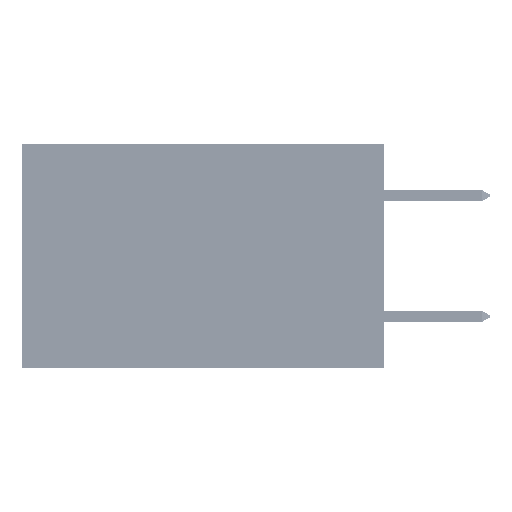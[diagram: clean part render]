
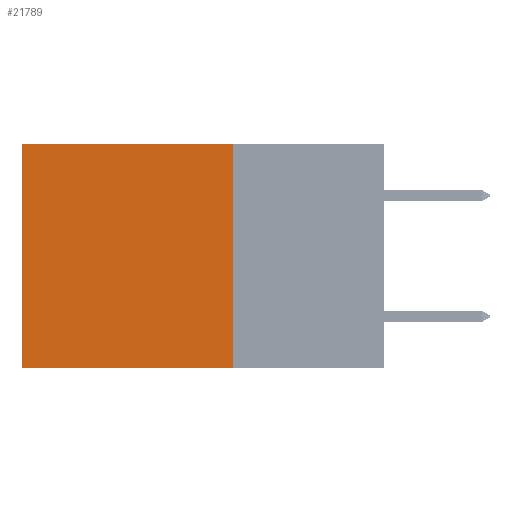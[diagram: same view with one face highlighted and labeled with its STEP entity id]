
A CAD part, left-side view. The second image highlights one B-rep face of the part: STEP entity #21789.
In plain terms, the highlighted planar face has unit normal (-1, 0, 0).
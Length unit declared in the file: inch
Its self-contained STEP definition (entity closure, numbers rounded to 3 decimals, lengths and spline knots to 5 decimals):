
#695 = ORIENTED_EDGE ( 'NONE', *, *, #42039, .T. ) ;
#1182 = VECTOR ( 'NONE', #9158, 39.37008 ) ;
#1398 = DIRECTION ( 'NONE',  ( 0., 1., 0. ) ) ;
#4452 = ORIENTED_EDGE ( 'NONE', *, *, #6993, .T. ) ;
#5292 = EDGE_CURVE ( 'NONE', #37169, #43508, #27434, .T. ) ;
#5573 = CARTESIAN_POINT ( 'NONE',  ( 0.2875, 0.25, 0. ) ) ;
#5742 = CARTESIAN_POINT ( 'NONE',  ( 0.2875, 0.25, 0. ) ) ;
#6723 = ORIENTED_EDGE ( 'NONE', *, *, #9416, .F. ) ;
#6993 = EDGE_CURVE ( 'NONE', #26703, #14465, #40642, .T. ) ;
#8527 = VECTOR ( 'NONE', #34752, 39.37008 ) ;
#8702 = DIRECTION ( 'NONE',  ( 0., 0., -1. ) ) ;
#8930 = LINE ( 'NONE', #22814, #25578 ) ;
#9158 = DIRECTION ( 'NONE',  ( 0., 0., -1. ) ) ;
#9416 = EDGE_CURVE ( 'NONE', #26703, #37169, #10590, .T. ) ;
#9745 = CARTESIAN_POINT ( 'NONE',  ( 0.2875, 0.25, -0.37 ) ) ;
#10570 = CARTESIAN_POINT ( 'NONE',  ( 0.2875, 0.6, 0. ) ) ;
#10590 = LINE ( 'NONE', #5573, #1182 ) ;
#12317 = VECTOR ( 'NONE', #1398, 39.37008 ) ;
#14465 = VERTEX_POINT ( 'NONE', #10570 ) ;
#20741 = ORIENTED_EDGE ( 'NONE', *, *, #5292, .F. ) ;
#21789 = ADVANCED_FACE ( 'NONE', ( #25027 ), #40375, .F. ) ;
#22814 = CARTESIAN_POINT ( 'NONE',  ( 0.2875, 0.6, 0. ) ) ;
#25027 = FACE_OUTER_BOUND ( 'NONE', #33649, .T. ) ;
#25578 = VECTOR ( 'NONE', #8702, 39.37008 ) ;
#26131 = DIRECTION ( 'NONE',  ( 1., 0., 0. ) ) ;
#26266 = CARTESIAN_POINT ( 'NONE',  ( 0.2875, 0.25, 0. ) ) ;
#26703 = VERTEX_POINT ( 'NONE', #5742 ) ;
#27075 = CARTESIAN_POINT ( 'NONE',  ( 0.2875, 0.6, -0.37 ) ) ;
#27434 = LINE ( 'NONE', #9745, #8527 ) ;
#29019 = CARTESIAN_POINT ( 'NONE',  ( 0.2875, 0.25, -0.37 ) ) ;
#30603 = AXIS2_PLACEMENT_3D ( 'NONE', #36819, #26131, #43946 ) ;
#33649 = EDGE_LOOP ( 'NONE', ( #695, #20741, #6723, #4452 ) ) ;
#34752 = DIRECTION ( 'NONE',  ( 0., 1., 0. ) ) ;
#36819 = CARTESIAN_POINT ( 'NONE',  ( 0.2875, 0.25, 0. ) ) ;
#37169 = VERTEX_POINT ( 'NONE', #29019 ) ;
#40375 = PLANE ( 'NONE',  #30603 ) ;
#40642 = LINE ( 'NONE', #26266, #12317 ) ;
#42039 = EDGE_CURVE ( 'NONE', #14465, #43508, #8930, .T. ) ;
#43508 = VERTEX_POINT ( 'NONE', #27075 ) ;
#43946 = DIRECTION ( 'NONE',  ( 0., 0., -1. ) ) ;
